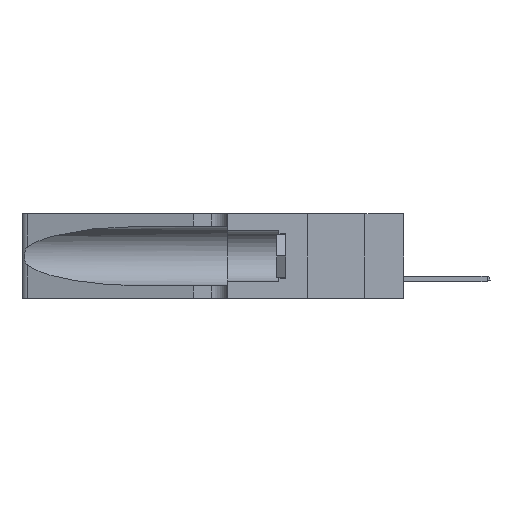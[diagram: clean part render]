
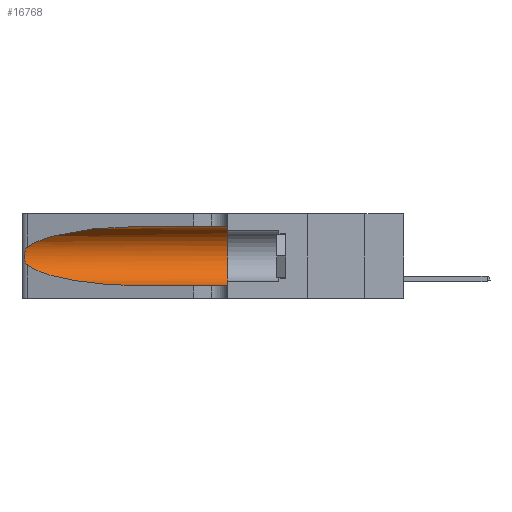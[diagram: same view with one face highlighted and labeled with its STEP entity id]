
A CAD part, left-side view. The second image highlights one B-rep face of the part: STEP entity #16768.
In plain terms, the highlighted cylindrical face has radius 3.308 mm (diameter 6.617 mm), a partial arc.
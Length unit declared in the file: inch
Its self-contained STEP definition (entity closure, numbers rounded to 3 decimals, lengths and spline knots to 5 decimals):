
#609 = CARTESIAN_POINT ( 'NONE',  ( 0.1305, 1.61858, 0.31525 ) ) ;
#842 = DIRECTION ( 'NONE',  ( 0., 0., -1. ) ) ;
#864 = CARTESIAN_POINT ( 'NONE',  ( 0.26075, 1.23896, 0.178 ) ) ;
#3639 = CARTESIAN_POINT ( 'NONE',  ( 0.1305, 0.72297, 0.31525 ) ) ;
#3798 = DIRECTION ( 'NONE',  ( 0., -1., 0. ) ) ;
#3818 = CARTESIAN_POINT ( 'NONE',  ( 0.25639, 1.23184, 0.21858 ) ) ;
#4091 = CARTESIAN_POINT ( 'NONE',  ( 0.25787, 1.23484, 0.2124 ) ) ;
#4386 = CARTESIAN_POINT ( 'NONE',  ( 0.25854, 1.2359, 0.20912 ) ) ;
#4389 = CARTESIAN_POINT ( 'NONE',  ( 0.25487, 1.22718, 0.22369 ) ) ;
#5333 = VECTOR ( 'NONE', #14311, 39.37008 ) ;
#5412 = CARTESIAN_POINT ( 'NONE',  ( 0.25639, 1.23186, 0.15144 ) ) ;
#5485 = VECTOR ( 'NONE', #37070, 39.37008 ) ;
#6326 = CARTESIAN_POINT ( 'NONE',  ( 0.25487, 1.22718, 0.14631 ) ) ;
#6917 =( BOUNDED_CURVE ( )  B_SPLINE_CURVE ( 3, ( #21944, #14434, #31657, #4389 ),
 .UNSPECIFIED., .F., .F. ) 
 B_SPLINE_CURVE_WITH_KNOTS ( ( 4, 4 ),
 ( 1.5708, 2.84003 ),
 .UNSPECIFIED. ) 
 CURVE ( )  GEOMETRIC_REPRESENTATION_ITEM ( )  RATIONAL_B_SPLINE_CURVE ( ( 1., 0.87, 0.87, 1. ) ) 
 REPRESENTATION_ITEM ( '' )  );
#7542 = AXIS2_PLACEMENT_3D ( 'NONE', #20755, #30793, #34194 ) ;
#7602 = CARTESIAN_POINT ( 'NONE',  ( 0.25856, 1.23593, 0.16098 ) ) ;
#8044 = CARTESIAN_POINT ( 'NONE',  ( 0.26018, 1.23835, 0.19895 ) ) ;
#9661 = CARTESIAN_POINT ( 'NONE',  ( 0.1305, 1.61858, 0.05475 ) ) ;
#9687 = VERTEX_POINT ( 'NONE', #27755 ) ;
#10427 = FACE_OUTER_BOUND ( 'NONE', #42598, .T. ) ;
#12416 = ORIENTED_EDGE ( 'NONE', *, *, #21689, .T. ) ;
#14311 = DIRECTION ( 'NONE',  ( 0., -1., 0. ) ) ;
#14434 = CARTESIAN_POINT ( 'NONE',  ( 0.18966, 0.96281, 0.31525 ) ) ;
#14540 = CARTESIAN_POINT ( 'NONE',  ( 0.1305, 0.35, 0.05475 ) ) ;
#15008 = EDGE_CURVE ( 'NONE', #31092, #16828, #6917, .T. ) ;
#16221 =( BOUNDED_CURVE ( )  B_SPLINE_CURVE ( 3, ( #6326, #33029, #39662, #16298 ),
 .UNSPECIFIED., .F., .T. ) 
 B_SPLINE_CURVE_WITH_KNOTS ( ( 4, 4 ),
 ( 3.44316, 4.71239 ),
 .UNSPECIFIED. ) 
 CURVE ( )  GEOMETRIC_REPRESENTATION_ITEM ( )  RATIONAL_B_SPLINE_CURVE ( ( 1., 0.87, 0.87, 1. ) ) 
 REPRESENTATION_ITEM ( '' )  );
#16298 = CARTESIAN_POINT ( 'NONE',  ( 0.1305, 0.72297, 0.05475 ) ) ;
#16475 = EDGE_CURVE ( 'NONE', #43416, #9687, #16221, .T. ) ;
#16768 = ADVANCED_FACE ( 'NONE', ( #10427 ), #20157, .F. ) ;
#16828 = VERTEX_POINT ( 'NONE', #27068 ) ;
#17665 = EDGE_CURVE ( 'NONE', #16828, #43416, #28708, .T. ) ;
#19147 = ORIENTED_EDGE ( 'NONE', *, *, #17665, .T. ) ;
#20124 = ORIENTED_EDGE ( 'NONE', *, *, #15008, .T. ) ;
#20157 = CYLINDRICAL_SURFACE ( 'NONE', #43764, 0.13025 ) ;
#20433 = ORIENTED_EDGE ( 'NONE', *, *, #40555, .F. ) ;
#20601 = CARTESIAN_POINT ( 'NONE',  ( 0.25487, 1.22718, 0.22369 ) ) ;
#20739 = CARTESIAN_POINT ( 'NONE',  ( 0.25555, 1.22994, 0.2215 ) ) ;
#20755 = CARTESIAN_POINT ( 'NONE',  ( 0.1305, 0.35, 0.185 ) ) ;
#21689 = EDGE_CURVE ( 'NONE', #9687, #28788, #21966, .T. ) ;
#21944 = CARTESIAN_POINT ( 'NONE',  ( 0.1305, 0.72297, 0.31525 ) ) ;
#21966 = LINE ( 'NONE', #9661, #5485 ) ;
#22385 = CARTESIAN_POINT ( 'NONE',  ( 0.25789, 1.23486, 0.15765 ) ) ;
#23028 = CIRCLE ( 'NONE', #7542, 0.13025 ) ;
#24302 = VERTEX_POINT ( 'NONE', #28184 ) ;
#24569 = CARTESIAN_POINT ( 'NONE',  ( 0.26017, 1.23833, 0.17102 ) ) ;
#27068 = CARTESIAN_POINT ( 'NONE',  ( 0.25487, 1.22718, 0.22369 ) ) ;
#27755 = CARTESIAN_POINT ( 'NONE',  ( 0.1305, 0.72297, 0.05475 ) ) ;
#28153 = EDGE_CURVE ( 'NONE', #24302, #28788, #23028, .T. ) ;
#28184 = CARTESIAN_POINT ( 'NONE',  ( 0.1305, 0.35, 0.31525 ) ) ;
#28708 = B_SPLINE_CURVE_WITH_KNOTS ( 'NONE', 3,
 ( #20601, #20739, #3818, #4091, #4386, #8044, #41379, #864, #24569, #7602, #22385, #5412, #39054, #35202 ),
 .UNSPECIFIED., .F., .F.,
 ( 4, 2, 2, 2, 2, 2, 4 ),
 ( 0., 0.00027, 0.00053, 0.00107, 0.0016, 0.00187, 0.00214 ),
 .UNSPECIFIED. ) ;
#28788 = VERTEX_POINT ( 'NONE', #14540 ) ;
#30793 = DIRECTION ( 'NONE',  ( 0., 1., 0. ) ) ;
#31092 = VERTEX_POINT ( 'NONE', #3639 ) ;
#31657 = CARTESIAN_POINT ( 'NONE',  ( 0.2373, 1.15595, 0.28018 ) ) ;
#33029 = CARTESIAN_POINT ( 'NONE',  ( 0.2373, 1.15595, 0.08982 ) ) ;
#34102 = CARTESIAN_POINT ( 'NONE',  ( 0.25487, 1.22718, 0.14631 ) ) ;
#34194 = DIRECTION ( 'NONE',  ( 0., 0., 1. ) ) ;
#34736 = CARTESIAN_POINT ( 'NONE',  ( 0.1305, 1.61858, 0.185 ) ) ;
#35011 = ORIENTED_EDGE ( 'NONE', *, *, #28153, .F. ) ;
#35202 = CARTESIAN_POINT ( 'NONE',  ( 0.25487, 1.22718, 0.14631 ) ) ;
#37070 = DIRECTION ( 'NONE',  ( 0., -1., 0. ) ) ;
#39054 = CARTESIAN_POINT ( 'NONE',  ( 0.25555, 1.22993, 0.14849 ) ) ;
#39271 = LINE ( 'NONE', #609, #5333 ) ;
#39662 = CARTESIAN_POINT ( 'NONE',  ( 0.18966, 0.96281, 0.05475 ) ) ;
#40555 = EDGE_CURVE ( 'NONE', #31092, #24302, #39271, .T. ) ;
#41379 = CARTESIAN_POINT ( 'NONE',  ( 0.26075, 1.23896, 0.19203 ) ) ;
#42598 = EDGE_LOOP ( 'NONE', ( #20124, #19147, #42650, #12416, #35011, #20433 ) ) ;
#42650 = ORIENTED_EDGE ( 'NONE', *, *, #16475, .T. ) ;
#43416 = VERTEX_POINT ( 'NONE', #34102 ) ;
#43764 = AXIS2_PLACEMENT_3D ( 'NONE', #34736, #3798, #842 ) ;
